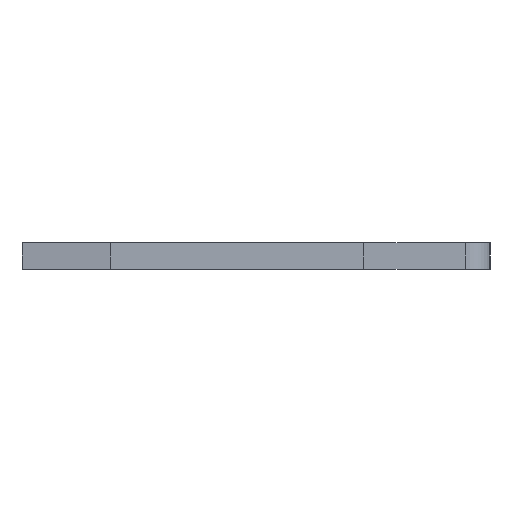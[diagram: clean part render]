
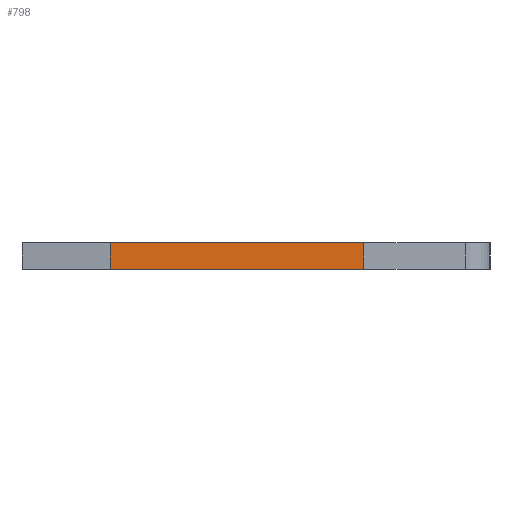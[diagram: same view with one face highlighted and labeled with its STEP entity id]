
A CAD part, left-side view. The second image highlights one B-rep face of the part: STEP entity #798.
In plain terms, the highlighted face is planar.
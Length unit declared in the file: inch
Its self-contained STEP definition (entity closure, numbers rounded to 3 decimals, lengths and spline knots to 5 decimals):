
#75 = CARTESIAN_POINT ( 'NONE',  ( 0.013, 0.146, -0.0575 ) ) ;
#88 = VECTOR ( 'NONE', #1501, 39.37008 ) ;
#143 = VERTEX_POINT ( 'NONE', #635 ) ;
#160 = VECTOR ( 'NONE', #1086, 39.37008 ) ;
#174 = CARTESIAN_POINT ( 'NONE',  ( -0.013, -0.099, -0.0575 ) ) ;
#242 = VECTOR ( 'NONE', #1571, 39.37008 ) ;
#422 = PLANE ( 'NONE',  #1407 ) ;
#433 = DIRECTION ( 'NONE',  ( 1., 0., 0. ) ) ;
#495 = LINE ( 'NONE', #1515, #160 ) ;
#535 = LINE ( 'NONE', #837, #88 ) ;
#635 = CARTESIAN_POINT ( 'NONE',  ( 0.013, 0.146, -0.0575 ) ) ;
#660 = CARTESIAN_POINT ( 'NONE',  ( 0.013, 0.146, -0.0575 ) ) ;
#732 = EDGE_CURVE ( 'NONE', #922, #1054, #535, .T. ) ;
#736 = ORIENTED_EDGE ( 'NONE', *, *, #961, .F. ) ;
#740 = EDGE_CURVE ( 'NONE', #934, #922, #495, .T. ) ;
#798 = ADVANCED_FACE ( 'NONE', ( #939 ), #422, .F. ) ;
#837 = CARTESIAN_POINT ( 'NONE',  ( -0.013, 0.146, -0.0575 ) ) ;
#851 = CARTESIAN_POINT ( 'NONE',  ( 0.013, -0.099, -0.0575 ) ) ;
#902 = DIRECTION ( 'NONE',  ( -1., 0., 0. ) ) ;
#922 = VERTEX_POINT ( 'NONE', #174 ) ;
#934 = VERTEX_POINT ( 'NONE', #851 ) ;
#939 = FACE_OUTER_BOUND ( 'NONE', #1138, .T. ) ;
#961 = EDGE_CURVE ( 'NONE', #934, #143, #1181, .T. ) ;
#1012 = ORIENTED_EDGE ( 'NONE', *, *, #732, .T. ) ;
#1020 = CARTESIAN_POINT ( 'NONE',  ( -0.013, 0.146, -0.0575 ) ) ;
#1027 = ORIENTED_EDGE ( 'NONE', *, *, #1209, .F. ) ;
#1054 = VERTEX_POINT ( 'NONE', #1020 ) ;
#1086 = DIRECTION ( 'NONE',  ( -1., 0., 0. ) ) ;
#1091 = DIRECTION ( 'NONE',  ( 0., 0., 1. ) ) ;
#1114 = ORIENTED_EDGE ( 'NONE', *, *, #740, .T. ) ;
#1138 = EDGE_LOOP ( 'NONE', ( #1012, #1027, #736, #1114 ) ) ;
#1181 = LINE ( 'NONE', #75, #242 ) ;
#1209 = EDGE_CURVE ( 'NONE', #143, #1054, #1615, .T. ) ;
#1213 = CARTESIAN_POINT ( 'NONE',  ( 0.013, 0.146, -0.0575 ) ) ;
#1407 = AXIS2_PLACEMENT_3D ( 'NONE', #1213, #1091, #433 ) ;
#1501 = DIRECTION ( 'NONE',  ( 0., 1., 0. ) ) ;
#1515 = CARTESIAN_POINT ( 'NONE',  ( 0.013, -0.099, -0.0575 ) ) ;
#1571 = DIRECTION ( 'NONE',  ( 0., 1., 0. ) ) ;
#1615 = LINE ( 'NONE', #660, #1661 ) ;
#1661 = VECTOR ( 'NONE', #902, 39.37008 ) ;
